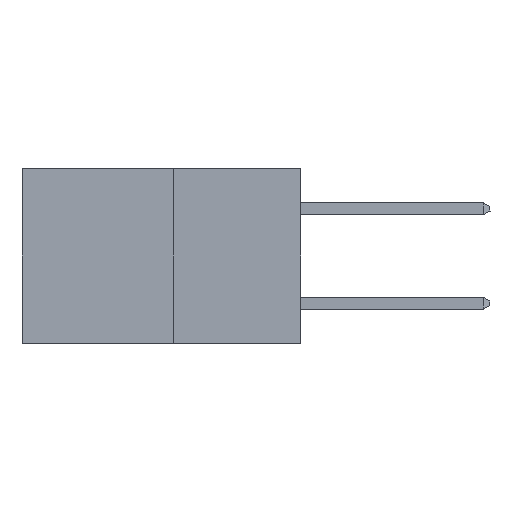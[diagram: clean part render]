
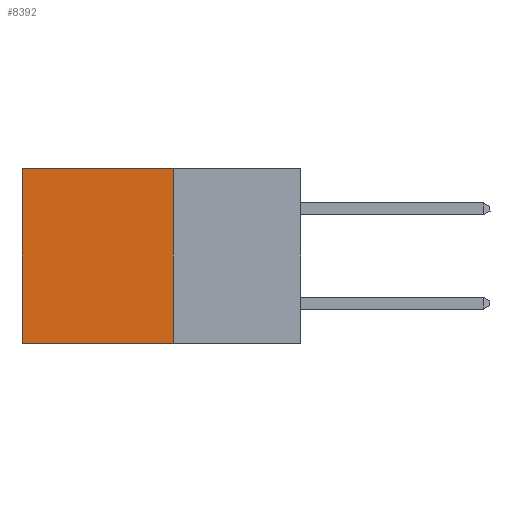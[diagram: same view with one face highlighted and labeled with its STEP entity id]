
A CAD part, left-side view. The second image highlights one B-rep face of the part: STEP entity #8392.
In plain terms, the highlighted planar face has unit normal (-1, 0, 0).
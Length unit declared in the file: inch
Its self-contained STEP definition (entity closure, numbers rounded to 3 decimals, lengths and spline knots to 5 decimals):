
#119 = VERTEX_POINT ( 'NONE', #17631 ) ;
#501 = VERTEX_POINT ( 'NONE', #7356 ) ;
#544 = DIRECTION ( 'NONE',  ( 0., 0., -1. ) ) ;
#1745 = VECTOR ( 'NONE', #18310, 39.37008 ) ;
#1960 = VECTOR ( 'NONE', #18212, 39.37008 ) ;
#2403 = EDGE_CURVE ( 'NONE', #7074, #8433, #5414, .T. ) ;
#2424 = LINE ( 'NONE', #9136, #1960 ) ;
#2681 = LINE ( 'NONE', #4555, #1745 ) ;
#4090 = LINE ( 'NONE', #8476, #11779 ) ;
#4555 = CARTESIAN_POINT ( 'NONE',  ( 0.277, 0.27, -0.37 ) ) ;
#5229 = ORIENTED_EDGE ( 'NONE', *, *, #2403, .T. ) ;
#5414 = LINE ( 'NONE', #12067, #8553 ) ;
#6030 = ORIENTED_EDGE ( 'NONE', *, *, #11370, .F. ) ;
#7074 = VERTEX_POINT ( 'NONE', #16973 ) ;
#7356 = CARTESIAN_POINT ( 'NONE',  ( 0.277, 0.59, -0.37 ) ) ;
#8267 = AXIS2_PLACEMENT_3D ( 'NONE', #15777, #9765, #544 ) ;
#8392 = ADVANCED_FACE ( 'NONE', ( #14312 ), #11211, .F. ) ;
#8433 = VERTEX_POINT ( 'NONE', #18886 ) ;
#8476 = CARTESIAN_POINT ( 'NONE',  ( 0.277, 0.59, -0.37 ) ) ;
#8553 = VECTOR ( 'NONE', #11590, 39.37008 ) ;
#9136 = CARTESIAN_POINT ( 'NONE',  ( 0.277, 0.27, -0.37 ) ) ;
#9765 = DIRECTION ( 'NONE',  ( 1., 0., 0. ) ) ;
#11211 = PLANE ( 'NONE',  #8267 ) ;
#11370 = EDGE_CURVE ( 'NONE', #119, #501, #2681, .T. ) ;
#11590 = DIRECTION ( 'NONE',  ( 0., 1., 0. ) ) ;
#11734 = EDGE_CURVE ( 'NONE', #8433, #501, #4090, .T. ) ;
#11779 = VECTOR ( 'NONE', #19095, 39.37008 ) ;
#12043 = EDGE_CURVE ( 'NONE', #7074, #119, #2424, .T. ) ;
#12067 = CARTESIAN_POINT ( 'NONE',  ( 0.277, 0.27, 0. ) ) ;
#14312 = FACE_OUTER_BOUND ( 'NONE', #19248, .T. ) ;
#14513 = ORIENTED_EDGE ( 'NONE', *, *, #12043, .F. ) ;
#15166 = ORIENTED_EDGE ( 'NONE', *, *, #11734, .T. ) ;
#15777 = CARTESIAN_POINT ( 'NONE',  ( 0.277, 0.27, -0.37 ) ) ;
#16973 = CARTESIAN_POINT ( 'NONE',  ( 0.277, 0.27, 0. ) ) ;
#17631 = CARTESIAN_POINT ( 'NONE',  ( 0.277, 0.27, -0.37 ) ) ;
#18212 = DIRECTION ( 'NONE',  ( 0., 0., -1. ) ) ;
#18310 = DIRECTION ( 'NONE',  ( 0., 1., 0. ) ) ;
#18886 = CARTESIAN_POINT ( 'NONE',  ( 0.277, 0.59, 0. ) ) ;
#19095 = DIRECTION ( 'NONE',  ( 0., 0., -1. ) ) ;
#19248 = EDGE_LOOP ( 'NONE', ( #15166, #6030, #14513, #5229 ) ) ;
